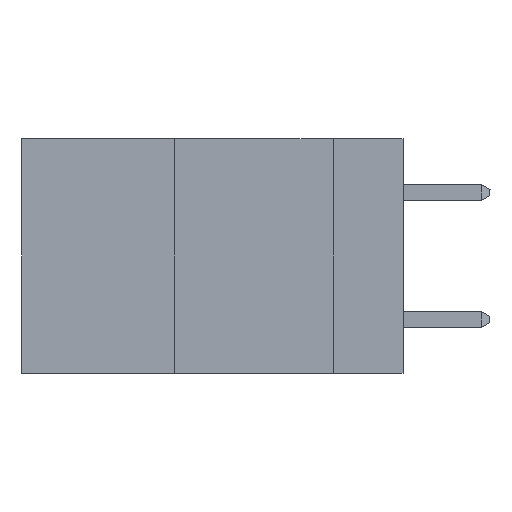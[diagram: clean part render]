
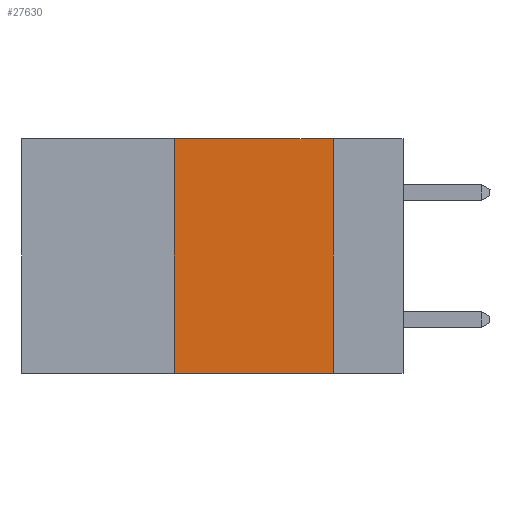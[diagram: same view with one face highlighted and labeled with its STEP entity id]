
A CAD part, left-side view. The second image highlights one B-rep face of the part: STEP entity #27630.
In plain terms, the highlighted planar face has unit normal (-1, 0, 0).
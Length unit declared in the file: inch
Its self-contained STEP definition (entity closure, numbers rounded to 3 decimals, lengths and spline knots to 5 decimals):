
#1033 = FACE_OUTER_BOUND ( 'NONE', #27410, .T. ) ;
#1446 = CARTESIAN_POINT ( 'NONE',  ( 0., 0.36, 0. ) ) ;
#1482 = LINE ( 'NONE', #1446, #27617 ) ;
#2314 = CARTESIAN_POINT ( 'NONE',  ( 0., 0.6, 0. ) ) ;
#2773 = VECTOR ( 'NONE', #10654, 39.37008 ) ;
#3228 = ORIENTED_EDGE ( 'NONE', *, *, #15212, .F. ) ;
#4712 = EDGE_CURVE ( 'NONE', #6093, #21127, #1482, .T. ) ;
#4725 = DIRECTION ( 'NONE',  ( 1., 0., 0. ) ) ;
#5892 = CARTESIAN_POINT ( 'NONE',  ( 0., 0.6, 0. ) ) ;
#5893 = EDGE_CURVE ( 'NONE', #21127, #17329, #21324, .T. ) ;
#6085 = DIRECTION ( 'NONE',  ( 0., -1., 0. ) ) ;
#6093 = VERTEX_POINT ( 'NONE', #17227 ) ;
#6200 = LINE ( 'NONE', #21278, #2773 ) ;
#6547 = DIRECTION ( 'NONE',  ( 0., 0., -1. ) ) ;
#10654 = DIRECTION ( 'NONE',  ( 0., -1., 0. ) ) ;
#10670 = EDGE_CURVE ( 'NONE', #6093, #13041, #6200, .T. ) ;
#13041 = VERTEX_POINT ( 'NONE', #17844 ) ;
#15212 = EDGE_CURVE ( 'NONE', #17329, #13041, #22824, .T. ) ;
#17227 = CARTESIAN_POINT ( 'NONE',  ( 0., 0.36, -0.37 ) ) ;
#17329 = VERTEX_POINT ( 'NONE', #21897 ) ;
#17844 = CARTESIAN_POINT ( 'NONE',  ( 0., 0.11, -0.37 ) ) ;
#18301 = AXIS2_PLACEMENT_3D ( 'NONE', #2314, #4725, #21907 ) ;
#18359 = VECTOR ( 'NONE', #6547, 39.37008 ) ;
#18666 = ORIENTED_EDGE ( 'NONE', *, *, #4712, .F. ) ;
#19004 = DIRECTION ( 'NONE',  ( 0., 0., 1. ) ) ;
#20067 = PLANE ( 'NONE',  #18301 ) ;
#21127 = VERTEX_POINT ( 'NONE', #22332 ) ;
#21278 = CARTESIAN_POINT ( 'NONE',  ( 0., 0.6, -0.37 ) ) ;
#21324 = LINE ( 'NONE', #5892, #26835 ) ;
#21897 = CARTESIAN_POINT ( 'NONE',  ( 0., 0.11, 0. ) ) ;
#21907 = DIRECTION ( 'NONE',  ( 0., 0., -1. ) ) ;
#22332 = CARTESIAN_POINT ( 'NONE',  ( 0., 0.36, 0. ) ) ;
#22685 = ORIENTED_EDGE ( 'NONE', *, *, #5893, .F. ) ;
#22824 = LINE ( 'NONE', #28269, #18359 ) ;
#26835 = VECTOR ( 'NONE', #6085, 39.37008 ) ;
#27410 = EDGE_LOOP ( 'NONE', ( #3228, #22685, #18666, #28343 ) ) ;
#27617 = VECTOR ( 'NONE', #19004, 39.37008 ) ;
#27630 = ADVANCED_FACE ( 'NONE', ( #1033 ), #20067, .F. ) ;
#28269 = CARTESIAN_POINT ( 'NONE',  ( 0., 0.11, 0. ) ) ;
#28343 = ORIENTED_EDGE ( 'NONE', *, *, #10670, .T. ) ;
